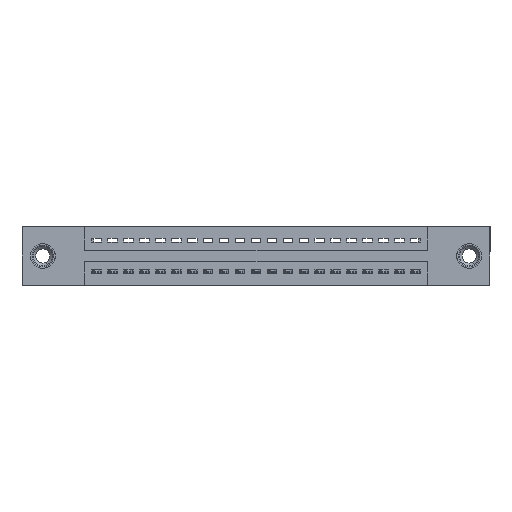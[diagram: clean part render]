
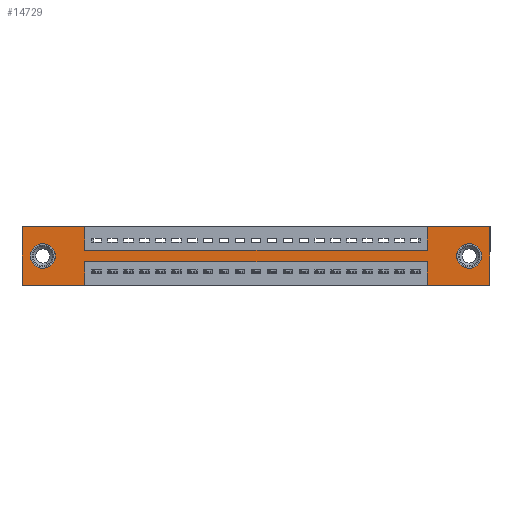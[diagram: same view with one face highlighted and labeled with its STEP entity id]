
A CAD part, front view. The second image highlights one B-rep face of the part: STEP entity #14729.
In plain terms, the highlighted planar face has unit normal (0, -1, 0).
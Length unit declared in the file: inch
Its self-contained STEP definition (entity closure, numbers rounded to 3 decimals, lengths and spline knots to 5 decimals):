
#119 = DIRECTION ( 'NONE',  ( 0., 0., -1. ) ) ;
#308 = DIRECTION ( 'NONE',  ( 0., 0., 1. ) ) ;
#352 = EDGE_CURVE ( 'NONE', #13705, #15509, #2638, .T. ) ;
#368 = CIRCLE ( 'NONE', #20663, 0.078 ) ;
#655 = LINE ( 'NONE', #6367, #3219 ) ;
#757 = VERTEX_POINT ( 'NONE', #18985 ) ;
#777 = ORIENTED_EDGE ( 'NONE', *, *, #4797, .F. ) ;
#812 = VECTOR ( 'NONE', #19878, 39.37008 ) ;
#814 = DIRECTION ( 'NONE',  ( 0., 0., -1. ) ) ;
#1124 = DIRECTION ( 'NONE',  ( 0., 1., 0. ) ) ;
#1352 = AXIS2_PLACEMENT_3D ( 'NONE', #6694, #9908, #308 ) ;
#1393 = FACE_BOUND ( 'NONE', #18003, .T. ) ;
#1568 = CARTESIAN_POINT ( 'NONE',  ( 0.3925, 0., -0.37 ) ) ;
#1611 = DIRECTION ( 'NONE',  ( -1., 0., 0. ) ) ;
#1655 = FACE_OUTER_BOUND ( 'NONE', #5694, .T. ) ;
#1776 = EDGE_CURVE ( 'NONE', #4155, #2767, #16638, .T. ) ;
#2320 = CARTESIAN_POINT ( 'NONE',  ( 2.805, 0., -0.185 ) ) ;
#2378 = VECTOR ( 'NONE', #15011, 39.37008 ) ;
#2446 = ORIENTED_EDGE ( 'NONE', *, *, #19810, .T. ) ;
#2575 = ORIENTED_EDGE ( 'NONE', *, *, #16027, .F. ) ;
#2638 = CIRCLE ( 'NONE', #1352, 0.078 ) ;
#2767 = VERTEX_POINT ( 'NONE', #7811 ) ;
#2812 = LINE ( 'NONE', #3144, #4824 ) ;
#3113 = EDGE_CURVE ( 'NONE', #9658, #17164, #2812, .T. ) ;
#3137 = EDGE_CURVE ( 'NONE', #20697, #17244, #15029, .T. ) ;
#3144 = CARTESIAN_POINT ( 'NONE',  ( 0., 0., 0. ) ) ;
#3219 = VECTOR ( 'NONE', #1611, 39.37008 ) ;
#3295 = VECTOR ( 'NONE', #16801, 39.37008 ) ;
#3564 = LINE ( 'NONE', #13900, #6530 ) ;
#3846 = VERTEX_POINT ( 'NONE', #15372 ) ;
#3910 = ORIENTED_EDGE ( 'NONE', *, *, #3113, .F. ) ;
#4155 = VERTEX_POINT ( 'NONE', #16802 ) ;
#4243 = CARTESIAN_POINT ( 'NONE',  ( 2.5425, 0., -0.15 ) ) ;
#4336 = VERTEX_POINT ( 'NONE', #4243 ) ;
#4435 = EDGE_CURVE ( 'NONE', #20385, #4155, #17751, .T. ) ;
#4797 = EDGE_CURVE ( 'NONE', #757, #4985, #5484, .T. ) ;
#4824 = VECTOR ( 'NONE', #7935, 39.37008 ) ;
#4839 = ORIENTED_EDGE ( 'NONE', *, *, #1776, .F. ) ;
#4850 = ORIENTED_EDGE ( 'NONE', *, *, #3137, .F. ) ;
#4985 = VERTEX_POINT ( 'NONE', #18341 ) ;
#5098 = CIRCLE ( 'NONE', #5359, 0.078 ) ;
#5347 = CARTESIAN_POINT ( 'NONE',  ( 0., 0., 0. ) ) ;
#5359 = AXIS2_PLACEMENT_3D ( 'NONE', #20499, #1124, #6035 ) ;
#5458 = CARTESIAN_POINT ( 'NONE',  ( 0.13, 0., -0.107 ) ) ;
#5484 = LINE ( 'NONE', #11953, #9697 ) ;
#5694 = EDGE_LOOP ( 'NONE', ( #4850, #17995, #4839, #11378, #17702, #777, #2575, #17303, #13725, #3910, #9885, #14512 ) ) ;
#5753 = CARTESIAN_POINT ( 'NONE',  ( 0.3925, 0., -0.37 ) ) ;
#5905 = CIRCLE ( 'NONE', #8437, 0.078 ) ;
#5929 = DIRECTION ( 'NONE',  ( 0., 1., 0. ) ) ;
#6014 = DIRECTION ( 'NONE',  ( 0., 0., -1. ) ) ;
#6035 = DIRECTION ( 'NONE',  ( 0., 0., 1. ) ) ;
#6249 = EDGE_LOOP ( 'NONE', ( #13415, #16323 ) ) ;
#6342 = CARTESIAN_POINT ( 'NONE',  ( 2.935, 0., -0.37 ) ) ;
#6360 = AXIS2_PLACEMENT_3D ( 'NONE', #16870, #16785, #814 ) ;
#6367 = CARTESIAN_POINT ( 'NONE',  ( 0., 0., -0.37 ) ) ;
#6494 = EDGE_CURVE ( 'NONE', #3846, #18566, #368, .T. ) ;
#6530 = VECTOR ( 'NONE', #6014, 39.37008 ) ;
#6694 = CARTESIAN_POINT ( 'NONE',  ( 0.13, 0., -0.185 ) ) ;
#6828 = LINE ( 'NONE', #8823, #812 ) ;
#7257 = PLANE ( 'NONE',  #6360 ) ;
#7564 = EDGE_CURVE ( 'NONE', #2767, #20697, #17933, .T. ) ;
#7736 = CARTESIAN_POINT ( 'NONE',  ( 0., 0., -0.37 ) ) ;
#7811 = CARTESIAN_POINT ( 'NONE',  ( 2.5425, 0., -0.22 ) ) ;
#7935 = DIRECTION ( 'NONE',  ( 1., 0., 0. ) ) ;
#8131 = VECTOR ( 'NONE', #19023, 39.37008 ) ;
#8212 = CARTESIAN_POINT ( 'NONE',  ( 0.3925, 0., -0.15 ) ) ;
#8437 = AXIS2_PLACEMENT_3D ( 'NONE', #2320, #16510, #10131 ) ;
#8534 = ORIENTED_EDGE ( 'NONE', *, *, #6494, .T. ) ;
#8594 = VECTOR ( 'NONE', #11935, 39.37008 ) ;
#8701 = CARTESIAN_POINT ( 'NONE',  ( 0., 0., -0.37 ) ) ;
#8794 = CARTESIAN_POINT ( 'NONE',  ( 2.5425, 0., 0. ) ) ;
#8823 = CARTESIAN_POINT ( 'NONE',  ( 0.3925, 0., -0.15 ) ) ;
#8931 = LINE ( 'NONE', #13502, #10192 ) ;
#9658 = VERTEX_POINT ( 'NONE', #9854 ) ;
#9697 = VECTOR ( 'NONE', #13493, 39.37008 ) ;
#9747 = EDGE_CURVE ( 'NONE', #14452, #9658, #18078, .T. ) ;
#9773 = CARTESIAN_POINT ( 'NONE',  ( 2.5425, 0., -0.37 ) ) ;
#9854 = CARTESIAN_POINT ( 'NONE',  ( 0., 0., 0. ) ) ;
#9885 = ORIENTED_EDGE ( 'NONE', *, *, #9747, .F. ) ;
#9908 = DIRECTION ( 'NONE',  ( 0., 1., 0. ) ) ;
#10131 = DIRECTION ( 'NONE',  ( 0., 0., -1. ) ) ;
#10192 = VECTOR ( 'NONE', #13486, 39.37008 ) ;
#10868 = LINE ( 'NONE', #8794, #8594 ) ;
#11063 = CARTESIAN_POINT ( 'NONE',  ( 0.3925, 0., -0.22 ) ) ;
#11378 = ORIENTED_EDGE ( 'NONE', *, *, #4435, .F. ) ;
#11935 = DIRECTION ( 'NONE',  ( 0., 0., 1. ) ) ;
#11953 = CARTESIAN_POINT ( 'NONE',  ( 0., 0., 0. ) ) ;
#12021 = VECTOR ( 'NONE', #14483, 39.37008 ) ;
#12289 = EDGE_CURVE ( 'NONE', #17244, #14452, #655, .T. ) ;
#13415 = ORIENTED_EDGE ( 'NONE', *, *, #16630, .T. ) ;
#13459 = VECTOR ( 'NONE', #16273, 39.37008 ) ;
#13486 = DIRECTION ( 'NONE',  ( 0., 0., -1. ) ) ;
#13493 = DIRECTION ( 'NONE',  ( 1., 0., 0. ) ) ;
#13502 = CARTESIAN_POINT ( 'NONE',  ( 2.935, 0., 0. ) ) ;
#13705 = VERTEX_POINT ( 'NONE', #14747 ) ;
#13725 = ORIENTED_EDGE ( 'NONE', *, *, #17385, .F. ) ;
#13900 = CARTESIAN_POINT ( 'NONE',  ( 0.3925, 0., 0. ) ) ;
#14316 = EDGE_CURVE ( 'NONE', #4985, #20385, #8931, .T. ) ;
#14452 = VERTEX_POINT ( 'NONE', #7736 ) ;
#14483 = DIRECTION ( 'NONE',  ( 0., 0., -1. ) ) ;
#14512 = ORIENTED_EDGE ( 'NONE', *, *, #12289, .F. ) ;
#14729 = ADVANCED_FACE ( 'NONE', ( #1393, #16184, #1655 ), #7257, .T. ) ;
#14747 = CARTESIAN_POINT ( 'NONE',  ( 0.13, 0., -0.263 ) ) ;
#15011 = DIRECTION ( 'NONE',  ( 0., 0., 1. ) ) ;
#15029 = LINE ( 'NONE', #1568, #12021 ) ;
#15244 = VERTEX_POINT ( 'NONE', #8212 ) ;
#15372 = CARTESIAN_POINT ( 'NONE',  ( 2.805, 0., -0.263 ) ) ;
#15509 = VERTEX_POINT ( 'NONE', #5458 ) ;
#16027 = EDGE_CURVE ( 'NONE', #4336, #757, #10868, .T. ) ;
#16184 = FACE_BOUND ( 'NONE', #6249, .T. ) ;
#16270 = CARTESIAN_POINT ( 'NONE',  ( 2.805, 0., -0.107 ) ) ;
#16273 = DIRECTION ( 'NONE',  ( -1., 0., 0. ) ) ;
#16323 = ORIENTED_EDGE ( 'NONE', *, *, #352, .T. ) ;
#16510 = DIRECTION ( 'NONE',  ( 0., 1., 0. ) ) ;
#16608 = EDGE_CURVE ( 'NONE', #15244, #4336, #6828, .T. ) ;
#16630 = EDGE_CURVE ( 'NONE', #15509, #13705, #5098, .T. ) ;
#16638 = LINE ( 'NONE', #9773, #2378 ) ;
#16785 = DIRECTION ( 'NONE',  ( 0., -1., 0. ) ) ;
#16801 = DIRECTION ( 'NONE',  ( 0., 0., 1. ) ) ;
#16802 = CARTESIAN_POINT ( 'NONE',  ( 2.5425, 0., -0.37 ) ) ;
#16870 = CARTESIAN_POINT ( 'NONE',  ( 0., 0., -0.37 ) ) ;
#17164 = VERTEX_POINT ( 'NONE', #18161 ) ;
#17166 = CARTESIAN_POINT ( 'NONE',  ( 0.3925, 0., -0.22 ) ) ;
#17244 = VERTEX_POINT ( 'NONE', #5753 ) ;
#17303 = ORIENTED_EDGE ( 'NONE', *, *, #16608, .F. ) ;
#17385 = EDGE_CURVE ( 'NONE', #17164, #15244, #3564, .T. ) ;
#17702 = ORIENTED_EDGE ( 'NONE', *, *, #14316, .F. ) ;
#17751 = LINE ( 'NONE', #8701, #13459 ) ;
#17933 = LINE ( 'NONE', #11063, #8131 ) ;
#17995 = ORIENTED_EDGE ( 'NONE', *, *, #7564, .F. ) ;
#18003 = EDGE_LOOP ( 'NONE', ( #2446, #8534 ) ) ;
#18078 = LINE ( 'NONE', #5347, #3295 ) ;
#18161 = CARTESIAN_POINT ( 'NONE',  ( 0.3925, 0., 0. ) ) ;
#18341 = CARTESIAN_POINT ( 'NONE',  ( 2.935, 0., 0. ) ) ;
#18566 = VERTEX_POINT ( 'NONE', #16270 ) ;
#18693 = CARTESIAN_POINT ( 'NONE',  ( 2.805, 0., -0.185 ) ) ;
#18985 = CARTESIAN_POINT ( 'NONE',  ( 2.5425, 0., 0. ) ) ;
#19023 = DIRECTION ( 'NONE',  ( -1., 0., 0. ) ) ;
#19810 = EDGE_CURVE ( 'NONE', #18566, #3846, #5905, .T. ) ;
#19878 = DIRECTION ( 'NONE',  ( 1., 0., 0. ) ) ;
#20385 = VERTEX_POINT ( 'NONE', #6342 ) ;
#20499 = CARTESIAN_POINT ( 'NONE',  ( 0.13, 0., -0.185 ) ) ;
#20663 = AXIS2_PLACEMENT_3D ( 'NONE', #18693, #5929, #119 ) ;
#20697 = VERTEX_POINT ( 'NONE', #17166 ) ;
